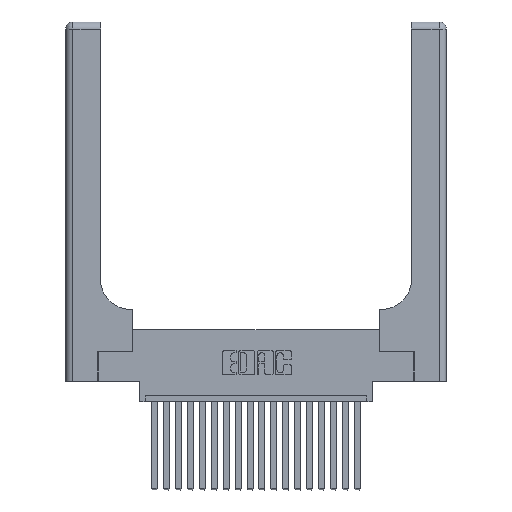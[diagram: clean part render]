
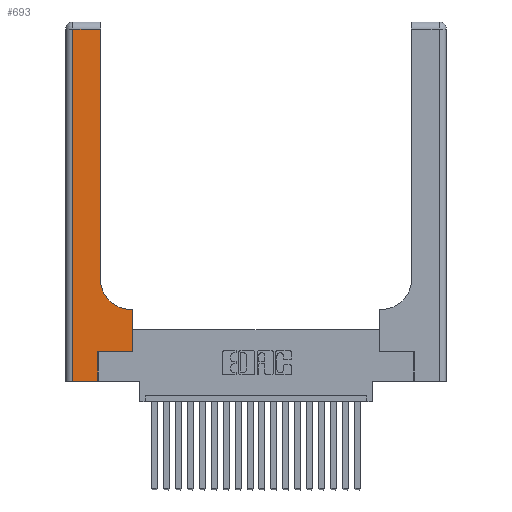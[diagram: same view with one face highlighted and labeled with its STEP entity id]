
A CAD part, top view. The second image highlights one B-rep face of the part: STEP entity #693.
In plain terms, the highlighted planar face has unit normal (0, 0, 1).
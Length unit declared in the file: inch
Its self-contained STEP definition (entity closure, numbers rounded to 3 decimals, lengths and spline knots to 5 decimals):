
#9 = CARTESIAN_POINT ( 'NONE',  ( 0.2915, 0.85, 0.37 ) ) ;
#478 = AXIS2_PLACEMENT_3D ( 'NONE', #18962, #10528, #705 ) ;
#693 = ADVANCED_FACE ( 'NONE', ( #13370 ), #13826, .F. ) ;
#705 = DIRECTION ( 'NONE',  ( -1., 0., 0. ) ) ;
#898 = LINE ( 'NONE', #6921, #18355 ) ;
#1072 = DIRECTION ( 'NONE',  ( 0., 0., -1. ) ) ;
#1560 = DIRECTION ( 'NONE',  ( -1., 0., 0. ) ) ;
#1753 = CARTESIAN_POINT ( 'NONE',  ( 0.2915, 0.6, 0.37 ) ) ;
#2207 = EDGE_CURVE ( 'NONE', #12895, #16476, #898, .T. ) ;
#2390 = EDGE_CURVE ( 'NONE', #16476, #17488, #5399, .T. ) ;
#2498 = VECTOR ( 'NONE', #15385, 39.37008 ) ;
#2865 = CARTESIAN_POINT ( 'NONE',  ( 0.269, 0.25, 0.37 ) ) ;
#2884 = DIRECTION ( 'NONE',  ( 1., 0., 0. ) ) ;
#3480 = DIRECTION ( 'NONE',  ( -1., 0., 0. ) ) ;
#3720 = ORIENTED_EDGE ( 'NONE', *, *, #16081, .T. ) ;
#4175 = ORIENTED_EDGE ( 'NONE', *, *, #15572, .T. ) ;
#4512 = LINE ( 'NONE', #20529, #15316 ) ;
#4911 = EDGE_CURVE ( 'NONE', #17488, #16629, #4512, .T. ) ;
#4968 = VECTOR ( 'NONE', #14623, 39.37008 ) ;
#4990 = VECTOR ( 'NONE', #13357, 39.37008 ) ;
#5399 = LINE ( 'NONE', #12017, #2498 ) ;
#5614 = LINE ( 'NONE', #14964, #11961 ) ;
#6307 = VERTEX_POINT ( 'NONE', #9 ) ;
#6710 = VECTOR ( 'NONE', #7482, 39.37008 ) ;
#6787 = ORIENTED_EDGE ( 'NONE', *, *, #2390, .T. ) ;
#6899 = EDGE_CURVE ( 'NONE', #6307, #15771, #16835, .T. ) ;
#6921 = CARTESIAN_POINT ( 'NONE',  ( 0.06, 3., 0.37 ) ) ;
#7354 = VERTEX_POINT ( 'NONE', #12838 ) ;
#7482 = DIRECTION ( 'NONE',  ( 0., 1., 0. ) ) ;
#7638 = CARTESIAN_POINT ( 'NONE',  ( 0.2915, 3., 0.37 ) ) ;
#7822 = CARTESIAN_POINT ( 'NONE',  ( 0.5415, 0.6, 0.37 ) ) ;
#8314 = ORIENTED_EDGE ( 'NONE', *, *, #12148, .T. ) ;
#9029 = CARTESIAN_POINT ( 'NONE',  ( 0.2915, 2.94, 0.37 ) ) ;
#10136 = EDGE_CURVE ( 'NONE', #15771, #12895, #5614, .T. ) ;
#10143 = CARTESIAN_POINT ( 'NONE',  ( 0.269, 0.25, 0.37 ) ) ;
#10229 = VERTEX_POINT ( 'NONE', #7822 ) ;
#10306 = VECTOR ( 'NONE', #3480, 39.37008 ) ;
#10528 = DIRECTION ( 'NONE',  ( 0., 0., -1. ) ) ;
#10953 = DIRECTION ( 'NONE',  ( 0., 1., 0. ) ) ;
#11170 = CARTESIAN_POINT ( 'NONE',  ( 0.5415, 0.85, 0.37 ) ) ;
#11961 = VECTOR ( 'NONE', #1560, 39.37008 ) ;
#12017 = CARTESIAN_POINT ( 'NONE',  ( 0., 0., 0.37 ) ) ;
#12148 = EDGE_CURVE ( 'NONE', #7354, #17627, #15623, .T. ) ;
#12578 = LINE ( 'NONE', #2865, #4968 ) ;
#12624 = EDGE_LOOP ( 'NONE', ( #15035, #15905, #14060, #6787, #15447, #3720, #8314, #20362, #4175 ) ) ;
#12838 = CARTESIAN_POINT ( 'NONE',  ( 0.5585, 0.25, 0.37 ) ) ;
#12895 = VERTEX_POINT ( 'NONE', #16727 ) ;
#13357 = DIRECTION ( 'NONE',  ( 0., 1., 0. ) ) ;
#13370 = FACE_OUTER_BOUND ( 'NONE', #12624, .T. ) ;
#13826 = PLANE ( 'NONE',  #478 ) ;
#13889 = EDGE_CURVE ( 'NONE', #17627, #10229, #14777, .T. ) ;
#14060 = ORIENTED_EDGE ( 'NONE', *, *, #2207, .T. ) ;
#14623 = DIRECTION ( 'NONE',  ( 1., 0., 0. ) ) ;
#14777 = LINE ( 'NONE', #1753, #10306 ) ;
#14964 = CARTESIAN_POINT ( 'NONE',  ( 0., 2.94, 0.37 ) ) ;
#15035 = ORIENTED_EDGE ( 'NONE', *, *, #6899, .T. ) ;
#15316 = VECTOR ( 'NONE', #10953, 39.37008 ) ;
#15385 = DIRECTION ( 'NONE',  ( 1., 0., 0. ) ) ;
#15447 = ORIENTED_EDGE ( 'NONE', *, *, #4911, .T. ) ;
#15572 = EDGE_CURVE ( 'NONE', #10229, #6307, #16024, .T. ) ;
#15623 = LINE ( 'NONE', #17563, #6710 ) ;
#15771 = VERTEX_POINT ( 'NONE', #9029 ) ;
#15905 = ORIENTED_EDGE ( 'NONE', *, *, #10136, .T. ) ;
#16024 = CIRCLE ( 'NONE', #17150, 0.25 ) ;
#16081 = EDGE_CURVE ( 'NONE', #16629, #7354, #12578, .T. ) ;
#16476 = VERTEX_POINT ( 'NONE', #18191 ) ;
#16629 = VERTEX_POINT ( 'NONE', #10143 ) ;
#16727 = CARTESIAN_POINT ( 'NONE',  ( 0.06, 2.94, 0.37 ) ) ;
#16835 = LINE ( 'NONE', #7638, #4990 ) ;
#17150 = AXIS2_PLACEMENT_3D ( 'NONE', #11170, #1072, #2884 ) ;
#17488 = VERTEX_POINT ( 'NONE', #20543 ) ;
#17563 = CARTESIAN_POINT ( 'NONE',  ( 0.5585, 0.25, 0.37 ) ) ;
#17606 = CARTESIAN_POINT ( 'NONE',  ( 0.5585, 0.6, 0.37 ) ) ;
#17627 = VERTEX_POINT ( 'NONE', #17606 ) ;
#18191 = CARTESIAN_POINT ( 'NONE',  ( 0.06, 0., 0.37 ) ) ;
#18355 = VECTOR ( 'NONE', #18725, 39.37008 ) ;
#18725 = DIRECTION ( 'NONE',  ( 0., -1., 0. ) ) ;
#18962 = CARTESIAN_POINT ( 'NONE',  ( 0., 3., 0.37 ) ) ;
#20362 = ORIENTED_EDGE ( 'NONE', *, *, #13889, .T. ) ;
#20529 = CARTESIAN_POINT ( 'NONE',  ( 0.269, 0., 0.37 ) ) ;
#20543 = CARTESIAN_POINT ( 'NONE',  ( 0.269, 0., 0.37 ) ) ;
